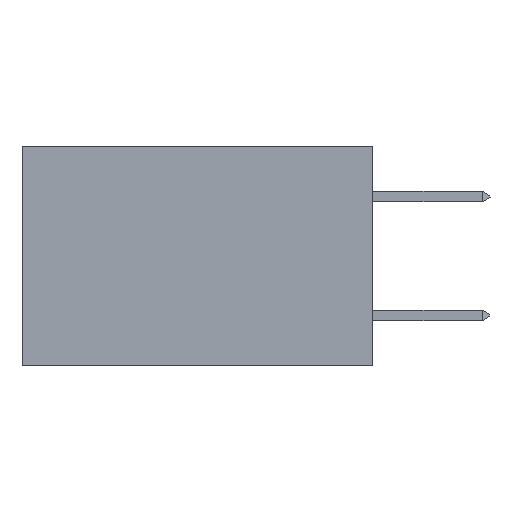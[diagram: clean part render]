
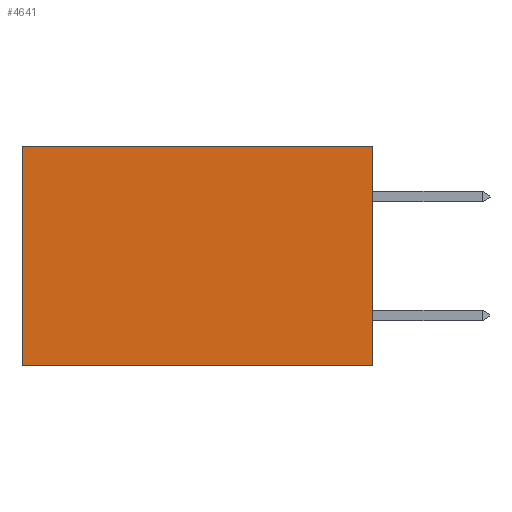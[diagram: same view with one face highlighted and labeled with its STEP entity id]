
A CAD part, left-side view. The second image highlights one B-rep face of the part: STEP entity #4641.
In plain terms, the highlighted planar face has unit normal (-1, 0, 0).
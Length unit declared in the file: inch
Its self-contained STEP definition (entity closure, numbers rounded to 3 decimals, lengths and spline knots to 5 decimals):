
#109 = DIRECTION ( 'NONE',  ( 0., 0., -1. ) ) ;
#222 = CARTESIAN_POINT ( 'NONE',  ( 0.277, 0., 0. ) ) ;
#434 = FACE_OUTER_BOUND ( 'NONE', #8169, .T. ) ;
#962 = VERTEX_POINT ( 'NONE', #4801 ) ;
#1048 = EDGE_CURVE ( 'NONE', #8907, #962, #7407, .T. ) ;
#1064 = EDGE_CURVE ( 'NONE', #9482, #8907, #8968, .T. ) ;
#1482 = EDGE_CURVE ( 'NONE', #9482, #5963, #8102, .T. ) ;
#1515 = CARTESIAN_POINT ( 'NONE',  ( 0.277, 0.59, 0. ) ) ;
#1619 = VECTOR ( 'NONE', #3924, 39.37008 ) ;
#2075 = AXIS2_PLACEMENT_3D ( 'NONE', #7165, #9185, #5027 ) ;
#2166 = EDGE_CURVE ( 'NONE', #5963, #962, #5810, .T. ) ;
#2473 = CARTESIAN_POINT ( 'NONE',  ( 0.277, 0.59, -0.37 ) ) ;
#3924 = DIRECTION ( 'NONE',  ( 0., 1., 0. ) ) ;
#4641 = ADVANCED_FACE ( 'NONE', ( #434 ), #8501, .F. ) ;
#4801 = CARTESIAN_POINT ( 'NONE',  ( 0.277, 0.59, -0.37 ) ) ;
#5027 = DIRECTION ( 'NONE',  ( 0., 0., -1. ) ) ;
#5063 = VECTOR ( 'NONE', #8028, 39.37008 ) ;
#5136 = CARTESIAN_POINT ( 'NONE',  ( 0.277, 0., -0.37 ) ) ;
#5810 = LINE ( 'NONE', #2473, #9233 ) ;
#5963 = VERTEX_POINT ( 'NONE', #1515 ) ;
#6007 = ORIENTED_EDGE ( 'NONE', *, *, #1048, .F. ) ;
#6032 = ORIENTED_EDGE ( 'NONE', *, *, #2166, .T. ) ;
#6619 = CARTESIAN_POINT ( 'NONE',  ( 0.277, 0., -0.37 ) ) ;
#7165 = CARTESIAN_POINT ( 'NONE',  ( 0.277, 0., -0.37 ) ) ;
#7190 = VECTOR ( 'NONE', #7735, 39.37008 ) ;
#7398 = ORIENTED_EDGE ( 'NONE', *, *, #1064, .F. ) ;
#7407 = LINE ( 'NONE', #8139, #7190 ) ;
#7444 = ORIENTED_EDGE ( 'NONE', *, *, #1482, .T. ) ;
#7735 = DIRECTION ( 'NONE',  ( 0., 1., 0. ) ) ;
#8028 = DIRECTION ( 'NONE',  ( 0., 0., -1. ) ) ;
#8102 = LINE ( 'NONE', #222, #1619 ) ;
#8139 = CARTESIAN_POINT ( 'NONE',  ( 0.277, 0., -0.37 ) ) ;
#8169 = EDGE_LOOP ( 'NONE', ( #6032, #6007, #7398, #7444 ) ) ;
#8501 = PLANE ( 'NONE',  #2075 ) ;
#8907 = VERTEX_POINT ( 'NONE', #5136 ) ;
#8968 = LINE ( 'NONE', #6619, #5063 ) ;
#9185 = DIRECTION ( 'NONE',  ( 1., 0., 0. ) ) ;
#9233 = VECTOR ( 'NONE', #109, 39.37008 ) ;
#9324 = CARTESIAN_POINT ( 'NONE',  ( 0.277, 0., 0. ) ) ;
#9482 = VERTEX_POINT ( 'NONE', #9324 ) ;
